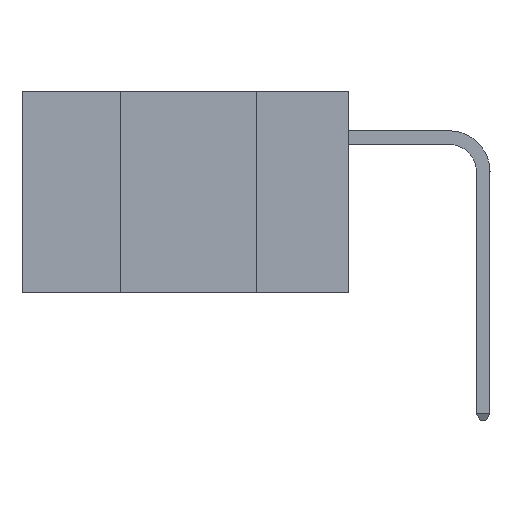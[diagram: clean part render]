
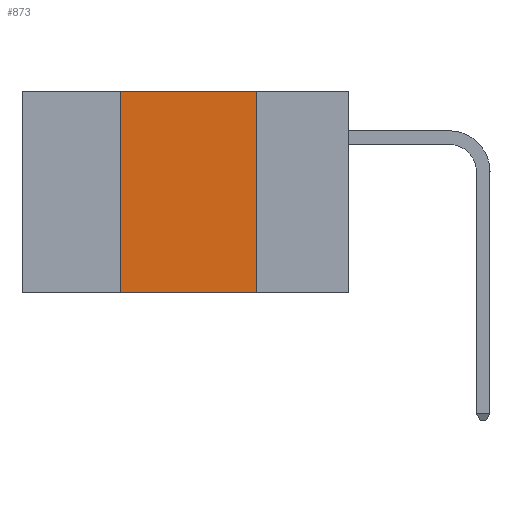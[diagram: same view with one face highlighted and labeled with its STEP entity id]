
A CAD part, left-side view. The second image highlights one B-rep face of the part: STEP entity #873.
In plain terms, the highlighted planar face has unit normal (-1, 0, 0).
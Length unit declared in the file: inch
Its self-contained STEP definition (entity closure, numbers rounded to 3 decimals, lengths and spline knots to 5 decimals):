
#822 = VERTEX_POINT ( 'NONE', #3290 ) ;
#873 = ADVANCED_FACE ( 'NONE', ( #1236 ), #5776, .F. ) ;
#925 = CARTESIAN_POINT ( 'NONE',  ( 0., 0.6, 0. ) ) ;
#1029 = DIRECTION ( 'NONE',  ( 0., 0., -1. ) ) ;
#1236 = FACE_OUTER_BOUND ( 'NONE', #7316, .T. ) ;
#1416 = LINE ( 'NONE', #13319, #13997 ) ;
#1769 = EDGE_CURVE ( 'NONE', #822, #8775, #5793, .T. ) ;
#1828 = DIRECTION ( 'NONE',  ( 0., -1., 0. ) ) ;
#3290 = CARTESIAN_POINT ( 'NONE',  ( 0., 0.17, 0. ) ) ;
#3787 = EDGE_CURVE ( 'NONE', #6863, #11333, #7384, .T. ) ;
#3813 = DIRECTION ( 'NONE',  ( 0., 0., -1. ) ) ;
#4266 = ORIENTED_EDGE ( 'NONE', *, *, #11390, .F. ) ;
#4355 = ORIENTED_EDGE ( 'NONE', *, *, #3787, .F. ) ;
#4561 = DIRECTION ( 'NONE',  ( 1., 0., 0. ) ) ;
#4576 = CARTESIAN_POINT ( 'NONE',  ( 0., 0.17, -0.37 ) ) ;
#5573 = LINE ( 'NONE', #10327, #7109 ) ;
#5776 = PLANE ( 'NONE',  #8947 ) ;
#5793 = LINE ( 'NONE', #8605, #10746 ) ;
#6147 = CARTESIAN_POINT ( 'NONE',  ( 0., 0.42, 0. ) ) ;
#6208 = CARTESIAN_POINT ( 'NONE',  ( 0., 0.42, -0.37 ) ) ;
#6863 = VERTEX_POINT ( 'NONE', #6208 ) ;
#7109 = VECTOR ( 'NONE', #1828, 39.37008 ) ;
#7316 = EDGE_LOOP ( 'NONE', ( #13258, #4266, #4355, #10271 ) ) ;
#7384 = LINE ( 'NONE', #12122, #10997 ) ;
#8605 = CARTESIAN_POINT ( 'NONE',  ( 0., 0.17, 0. ) ) ;
#8775 = VERTEX_POINT ( 'NONE', #4576 ) ;
#8947 = AXIS2_PLACEMENT_3D ( 'NONE', #925, #4561, #1029 ) ;
#10271 = ORIENTED_EDGE ( 'NONE', *, *, #13718, .T. ) ;
#10327 = CARTESIAN_POINT ( 'NONE',  ( 0., 0.6, -0.37 ) ) ;
#10746 = VECTOR ( 'NONE', #3813, 39.37008 ) ;
#10997 = VECTOR ( 'NONE', #11047, 39.37008 ) ;
#11047 = DIRECTION ( 'NONE',  ( 0., 0., 1. ) ) ;
#11333 = VERTEX_POINT ( 'NONE', #6147 ) ;
#11390 = EDGE_CURVE ( 'NONE', #11333, #822, #1416, .T. ) ;
#12122 = CARTESIAN_POINT ( 'NONE',  ( 0., 0.42, 0. ) ) ;
#13258 = ORIENTED_EDGE ( 'NONE', *, *, #1769, .F. ) ;
#13319 = CARTESIAN_POINT ( 'NONE',  ( 0., 0.6, 0. ) ) ;
#13718 = EDGE_CURVE ( 'NONE', #6863, #8775, #5573, .T. ) ;
#13913 = DIRECTION ( 'NONE',  ( 0., -1., 0. ) ) ;
#13997 = VECTOR ( 'NONE', #13913, 39.37008 ) ;
